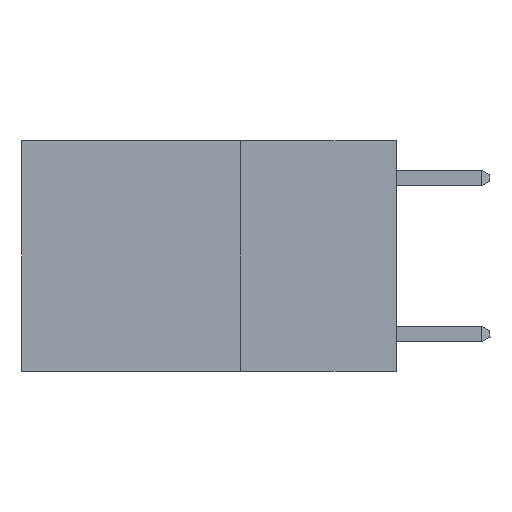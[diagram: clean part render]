
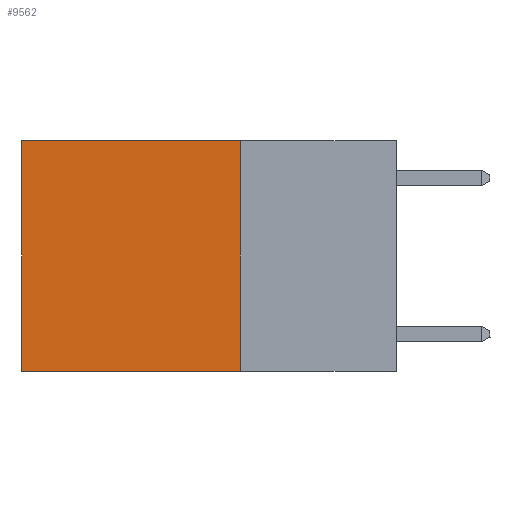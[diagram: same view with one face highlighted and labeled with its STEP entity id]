
A CAD part, left-side view. The second image highlights one B-rep face of the part: STEP entity #9562.
In plain terms, the highlighted planar face has unit normal (-1, 0, 0).
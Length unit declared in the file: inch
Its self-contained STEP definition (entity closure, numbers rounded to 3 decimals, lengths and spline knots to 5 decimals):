
#168 = ORIENTED_EDGE ( 'NONE', *, *, #6416, .T. ) ;
#1406 = VERTEX_POINT ( 'NONE', #16951 ) ;
#1552 = LINE ( 'NONE', #11501, #11782 ) ;
#1768 = PLANE ( 'NONE',  #15827 ) ;
#1891 = LINE ( 'NONE', #11655, #12772 ) ;
#1921 = EDGE_CURVE ( 'NONE', #15700, #9336, #1891, .T. ) ;
#2055 = DIRECTION ( 'NONE',  ( 0., 0., -1. ) ) ;
#2093 = ORIENTED_EDGE ( 'NONE', *, *, #12602, .T. ) ;
#3562 = VECTOR ( 'NONE', #5415, 39.37008 ) ;
#4211 = ORIENTED_EDGE ( 'NONE', *, *, #14536, .F. ) ;
#4790 = DIRECTION ( 'NONE',  ( 1., 0., 0. ) ) ;
#5415 = DIRECTION ( 'NONE',  ( 0., 0., -1. ) ) ;
#6416 = EDGE_CURVE ( 'NONE', #1406, #9863, #6600, .T. ) ;
#6600 = LINE ( 'NONE', #6777, #16178 ) ;
#6777 = CARTESIAN_POINT ( 'NONE',  ( 0.2625, 0.25, 0. ) ) ;
#8168 = CARTESIAN_POINT ( 'NONE',  ( 0.2625, 0.25, -0.37 ) ) ;
#8494 = DIRECTION ( 'NONE',  ( 0., 0., -1. ) ) ;
#8605 = ORIENTED_EDGE ( 'NONE', *, *, #1921, .F. ) ;
#9336 = VERTEX_POINT ( 'NONE', #12655 ) ;
#9562 = ADVANCED_FACE ( 'NONE', ( #11832 ), #1768, .F. ) ;
#9863 = VERTEX_POINT ( 'NONE', #13915 ) ;
#10459 = DIRECTION ( 'NONE',  ( 0., 1., 0. ) ) ;
#10896 = LINE ( 'NONE', #16459, #3562 ) ;
#11501 = CARTESIAN_POINT ( 'NONE',  ( 0.2625, 0.25, 0. ) ) ;
#11544 = CARTESIAN_POINT ( 'NONE',  ( 0.2625, 0.25, 0. ) ) ;
#11655 = CARTESIAN_POINT ( 'NONE',  ( 0.2625, 0.25, -0.37 ) ) ;
#11782 = VECTOR ( 'NONE', #8494, 39.37008 ) ;
#11832 = FACE_OUTER_BOUND ( 'NONE', #15326, .T. ) ;
#12602 = EDGE_CURVE ( 'NONE', #9863, #9336, #10896, .T. ) ;
#12655 = CARTESIAN_POINT ( 'NONE',  ( 0.2625, 0.6, -0.37 ) ) ;
#12772 = VECTOR ( 'NONE', #10459, 39.37008 ) ;
#13915 = CARTESIAN_POINT ( 'NONE',  ( 0.2625, 0.6, 0. ) ) ;
#14536 = EDGE_CURVE ( 'NONE', #1406, #15700, #1552, .T. ) ;
#14824 = DIRECTION ( 'NONE',  ( 0., 1., 0. ) ) ;
#15326 = EDGE_LOOP ( 'NONE', ( #2093, #8605, #4211, #168 ) ) ;
#15700 = VERTEX_POINT ( 'NONE', #8168 ) ;
#15827 = AXIS2_PLACEMENT_3D ( 'NONE', #11544, #4790, #2055 ) ;
#16178 = VECTOR ( 'NONE', #14824, 39.37008 ) ;
#16459 = CARTESIAN_POINT ( 'NONE',  ( 0.2625, 0.6, 0. ) ) ;
#16951 = CARTESIAN_POINT ( 'NONE',  ( 0.2625, 0.25, 0. ) ) ;
